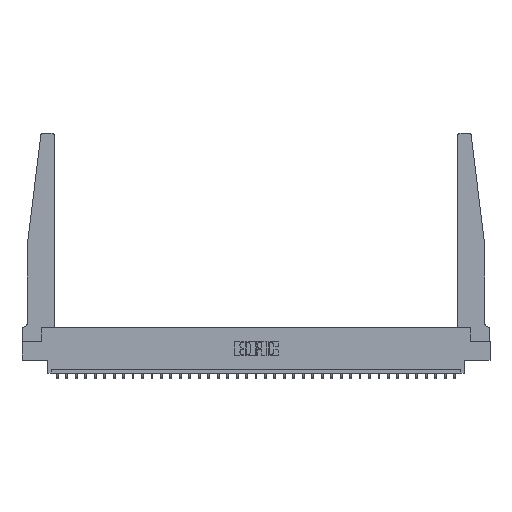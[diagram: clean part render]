
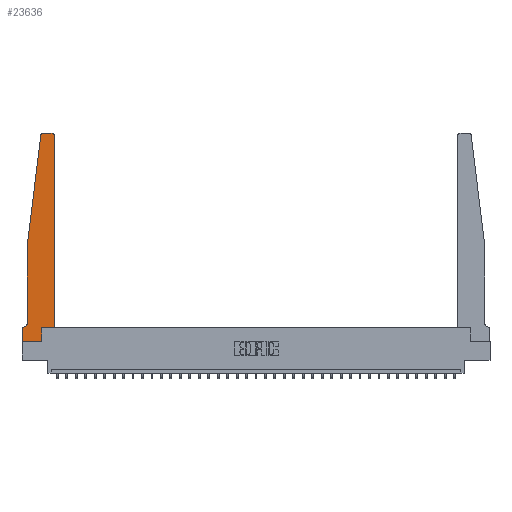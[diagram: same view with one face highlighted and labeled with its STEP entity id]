
A CAD part, top view. The second image highlights one B-rep face of the part: STEP entity #23636.
In plain terms, the highlighted planar face has unit normal (0, 0, 1).
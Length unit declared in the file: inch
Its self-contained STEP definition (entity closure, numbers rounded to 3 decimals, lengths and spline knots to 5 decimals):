
#212 = DIRECTION ( 'NONE',  ( 1., 0., 0. ) ) ;
#243 = DIRECTION ( 'NONE',  ( 0., 0., -1. ) ) ;
#420 = VECTOR ( 'NONE', #29848, 39.37008 ) ;
#423 = LINE ( 'NONE', #20083, #30273 ) ;
#661 = CARTESIAN_POINT ( 'NONE',  ( 0.425, 0.18, 0.37 ) ) ;
#967 = ORIENTED_EDGE ( 'NONE', *, *, #27025, .T. ) ;
#1084 = VERTEX_POINT ( 'NONE', #14545 ) ;
#1763 = EDGE_CURVE ( 'NONE', #7879, #30252, #12405, .T. ) ;
#2067 = ORIENTED_EDGE ( 'NONE', *, *, #3994, .T. ) ;
#2142 = CARTESIAN_POINT ( 'NONE',  ( 0.2605, 0., 0.37 ) ) ;
#2406 = PLANE ( 'NONE',  #9217 ) ;
#2557 = EDGE_CURVE ( 'NONE', #13951, #6116, #423, .T. ) ;
#2709 = CARTESIAN_POINT ( 'NONE',  ( 0.065, 0.2375, 0.37 ) ) ;
#2819 = DIRECTION ( 'NONE',  ( -1., 0., 0. ) ) ;
#3421 = CIRCLE ( 'NONE', #18865, 0.05 ) ;
#3994 = EDGE_CURVE ( 'NONE', #6116, #9140, #30057, .T. ) ;
#4215 = EDGE_CURVE ( 'NONE', #1084, #19826, #13000, .T. ) ;
#4879 = ORIENTED_EDGE ( 'NONE', *, *, #30678, .T. ) ;
#5270 = CARTESIAN_POINT ( 'NONE',  ( 0.395, 2.75, 0.37 ) ) ;
#5318 = DIRECTION ( 'NONE',  ( 0., 1., 0. ) ) ;
#5741 = CARTESIAN_POINT ( 'NONE',  ( 0., 0., 0.37 ) ) ;
#6116 = VERTEX_POINT ( 'NONE', #16032 ) ;
#6452 = DIRECTION ( 'NONE',  ( 0., -1., 0. ) ) ;
#6572 = VECTOR ( 'NONE', #6452, 39.37008 ) ;
#6950 = LINE ( 'NONE', #9380, #26733 ) ;
#7014 = EDGE_CURVE ( 'NONE', #9140, #18244, #11250, .T. ) ;
#7496 = CARTESIAN_POINT ( 'NONE',  ( 0.27653, 2.72, 0.37 ) ) ;
#7879 = VERTEX_POINT ( 'NONE', #18612 ) ;
#8589 = CARTESIAN_POINT ( 'NONE',  ( 0.065, 0.1875, 0.37 ) ) ;
#8723 = LINE ( 'NONE', #26064, #6572 ) ;
#9140 = VERTEX_POINT ( 'NONE', #17982 ) ;
#9217 = AXIS2_PLACEMENT_3D ( 'NONE', #29580, #24049, #22890 ) ;
#9301 = EDGE_CURVE ( 'NONE', #19826, #17675, #6950, .T. ) ;
#9380 = CARTESIAN_POINT ( 'NONE',  ( 0., 0., 0.37 ) ) ;
#9696 = EDGE_LOOP ( 'NONE', ( #14049, #2067, #20920, #26780, #22084, #19925, #27585, #11535, #24887, #4879, #18585, #967 ) ) ;
#9726 = CARTESIAN_POINT ( 'NONE',  ( 0.2605, 0.18, 0.37 ) ) ;
#10847 = VECTOR ( 'NONE', #212, 39.37008 ) ;
#11250 = LINE ( 'NONE', #18065, #20259 ) ;
#11535 = ORIENTED_EDGE ( 'NONE', *, *, #9301, .T. ) ;
#11615 = EDGE_CURVE ( 'NONE', #18244, #14051, #8723, .T. ) ;
#11878 = DIRECTION ( 'NONE',  ( 0., 0., 1. ) ) ;
#12405 = LINE ( 'NONE', #661, #17793 ) ;
#12482 = CARTESIAN_POINT ( 'NONE',  ( 0.425, 2.72, 0.37 ) ) ;
#12652 = CARTESIAN_POINT ( 'NONE',  ( 0.015, 0.1875, 0.37 ) ) ;
#12677 = DIRECTION ( 'NONE',  ( 0., -1., 0. ) ) ;
#13000 = LINE ( 'NONE', #5741, #23700 ) ;
#13285 = LINE ( 'NONE', #8589, #23555 ) ;
#13951 = VERTEX_POINT ( 'NONE', #5270 ) ;
#14049 = ORIENTED_EDGE ( 'NONE', *, *, #2557, .T. ) ;
#14051 = VERTEX_POINT ( 'NONE', #2709 ) ;
#14545 = CARTESIAN_POINT ( 'NONE',  ( 0., 0.1875, 0.37 ) ) ;
#14559 = CARTESIAN_POINT ( 'NONE',  ( 0.395, 2.72, 0.37 ) ) ;
#14830 = AXIS2_PLACEMENT_3D ( 'NONE', #7496, #11878, #19304 ) ;
#14885 = DIRECTION ( 'NONE',  ( 1., 0., 0. ) ) ;
#15381 = CARTESIAN_POINT ( 'NONE',  ( 0.2605, 0.18, 0.37 ) ) ;
#15494 = AXIS2_PLACEMENT_3D ( 'NONE', #14559, #21853, #14885 ) ;
#16032 = CARTESIAN_POINT ( 'NONE',  ( 0.27653, 2.75, 0.37 ) ) ;
#17675 = VERTEX_POINT ( 'NONE', #2142 ) ;
#17793 = VECTOR ( 'NONE', #5318, 39.37008 ) ;
#17982 = CARTESIAN_POINT ( 'NONE',  ( 0.24675, 2.72367, 0.37 ) ) ;
#18065 = CARTESIAN_POINT ( 'NONE',  ( 0.065, 1.25, 0.37 ) ) ;
#18244 = VERTEX_POINT ( 'NONE', #22750 ) ;
#18585 = ORIENTED_EDGE ( 'NONE', *, *, #1763, .T. ) ;
#18612 = CARTESIAN_POINT ( 'NONE',  ( 0.425, 0.18, 0.37 ) ) ;
#18865 = AXIS2_PLACEMENT_3D ( 'NONE', #19745, #243, #2819 ) ;
#19106 = EDGE_CURVE ( 'NONE', #14051, #22879, #3421, .T. ) ;
#19246 = DIRECTION ( 'NONE',  ( 1., 0., 0. ) ) ;
#19304 = DIRECTION ( 'NONE',  ( 1., 0., 0. ) ) ;
#19745 = CARTESIAN_POINT ( 'NONE',  ( 0.015, 0.2375, 0.37 ) ) ;
#19826 = VERTEX_POINT ( 'NONE', #22719 ) ;
#19923 = DIRECTION ( 'NONE',  ( -1., 0., 0. ) ) ;
#19925 = ORIENTED_EDGE ( 'NONE', *, *, #20414, .T. ) ;
#20083 = CARTESIAN_POINT ( 'NONE',  ( 0.25, 2.75, 0.37 ) ) ;
#20259 = VECTOR ( 'NONE', #30413, 39.37008 ) ;
#20414 = EDGE_CURVE ( 'NONE', #22879, #1084, #13285, .T. ) ;
#20679 = CIRCLE ( 'NONE', #15494, 0.03 ) ;
#20920 = ORIENTED_EDGE ( 'NONE', *, *, #7014, .T. ) ;
#21120 = EDGE_CURVE ( 'NONE', #17675, #31503, #26339, .T. ) ;
#21853 = DIRECTION ( 'NONE',  ( 0., 0., 1. ) ) ;
#22084 = ORIENTED_EDGE ( 'NONE', *, *, #19106, .T. ) ;
#22312 = CARTESIAN_POINT ( 'NONE',  ( 0.425, 0.18, 0.37 ) ) ;
#22719 = CARTESIAN_POINT ( 'NONE',  ( 0., 0., 0.37 ) ) ;
#22750 = CARTESIAN_POINT ( 'NONE',  ( 0.065, 1.25, 0.37 ) ) ;
#22879 = VERTEX_POINT ( 'NONE', #12652 ) ;
#22890 = DIRECTION ( 'NONE',  ( 1., 0., 0. ) ) ;
#23555 = VECTOR ( 'NONE', #30956, 39.37008 ) ;
#23636 = ADVANCED_FACE ( 'NONE', ( #24520 ), #2406, .T. ) ;
#23700 = VECTOR ( 'NONE', #12677, 39.37008 ) ;
#24049 = DIRECTION ( 'NONE',  ( 0., 0., 1. ) ) ;
#24520 = FACE_OUTER_BOUND ( 'NONE', #9696, .T. ) ;
#24887 = ORIENTED_EDGE ( 'NONE', *, *, #21120, .T. ) ;
#26064 = CARTESIAN_POINT ( 'NONE',  ( 0.065, 1.25, 0.37 ) ) ;
#26339 = LINE ( 'NONE', #9726, #420 ) ;
#26733 = VECTOR ( 'NONE', #19246, 39.37008 ) ;
#26780 = ORIENTED_EDGE ( 'NONE', *, *, #11615, .T. ) ;
#27025 = EDGE_CURVE ( 'NONE', #30252, #13951, #20679, .T. ) ;
#27585 = ORIENTED_EDGE ( 'NONE', *, *, #4215, .T. ) ;
#29324 = LINE ( 'NONE', #22312, #10847 ) ;
#29580 = CARTESIAN_POINT ( 'NONE',  ( 0., 0.1875, 0.37 ) ) ;
#29848 = DIRECTION ( 'NONE',  ( 0., 1., 0. ) ) ;
#30057 = CIRCLE ( 'NONE', #14830, 0.03 ) ;
#30252 = VERTEX_POINT ( 'NONE', #12482 ) ;
#30273 = VECTOR ( 'NONE', #19923, 39.37008 ) ;
#30413 = DIRECTION ( 'NONE',  ( -0.122, -0.992, 0. ) ) ;
#30678 = EDGE_CURVE ( 'NONE', #31503, #7879, #29324, .T. ) ;
#30956 = DIRECTION ( 'NONE',  ( -1., 0., 0. ) ) ;
#31503 = VERTEX_POINT ( 'NONE', #15381 ) ;
